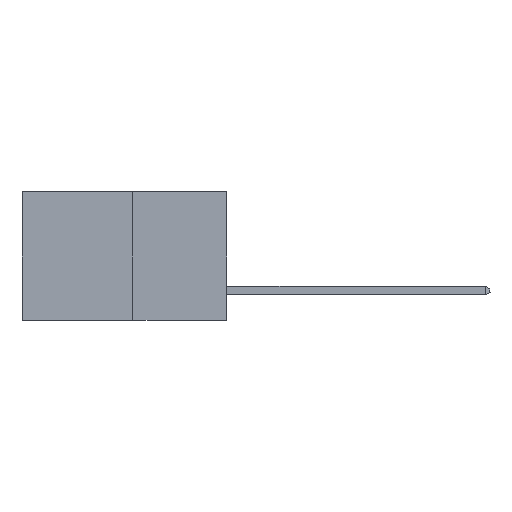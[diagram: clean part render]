
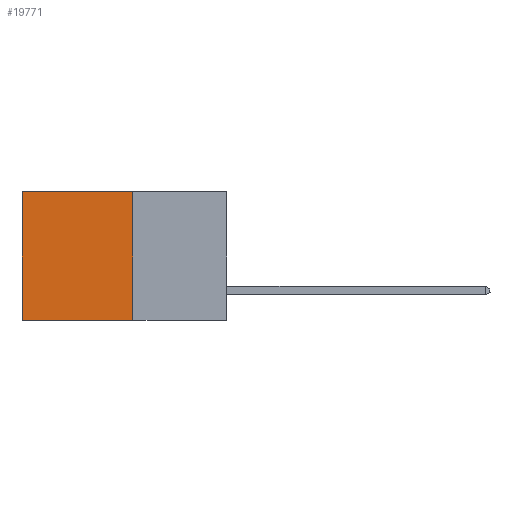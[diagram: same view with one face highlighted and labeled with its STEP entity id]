
A CAD part, left-side view. The second image highlights one B-rep face of the part: STEP entity #19771.
In plain terms, the highlighted planar face has unit normal (-1, 0, 0).
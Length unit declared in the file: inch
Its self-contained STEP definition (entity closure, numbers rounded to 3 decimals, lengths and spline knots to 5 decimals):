
#336 = EDGE_CURVE ( 'NONE', #10255, #24896, #18124, .T. ) ;
#1168 = EDGE_CURVE ( 'NONE', #4737, #10255, #10247, .T. ) ;
#2337 = CARTESIAN_POINT ( 'NONE',  ( 0.277, 0.59, 0. ) ) ;
#2595 = EDGE_CURVE ( 'NONE', #4737, #15701, #15443, .T. ) ;
#3167 = VECTOR ( 'NONE', #24520, 39.37008 ) ;
#3870 = LINE ( 'NONE', #15518, #3167 ) ;
#4200 = CARTESIAN_POINT ( 'NONE',  ( 0.277, 0.59, -0.37 ) ) ;
#4737 = VERTEX_POINT ( 'NONE', #5596 ) ;
#5028 = DIRECTION ( 'NONE',  ( 0., 1., 0. ) ) ;
#5182 = CARTESIAN_POINT ( 'NONE',  ( 0.277, 0.27, -0.37 ) ) ;
#5596 = CARTESIAN_POINT ( 'NONE',  ( 0.277, 0.27, 0. ) ) ;
#7398 = DIRECTION ( 'NONE',  ( 0., 0., -1. ) ) ;
#8435 = CARTESIAN_POINT ( 'NONE',  ( 0.277, 0.59, -0.37 ) ) ;
#9461 = VECTOR ( 'NONE', #16624, 39.37008 ) ;
#10025 = AXIS2_PLACEMENT_3D ( 'NONE', #5182, #20861, #7398 ) ;
#10247 = LINE ( 'NONE', #17994, #28091 ) ;
#10255 = VERTEX_POINT ( 'NONE', #2337 ) ;
#11436 = VECTOR ( 'NONE', #26045, 39.37008 ) ;
#13167 = ORIENTED_EDGE ( 'NONE', *, *, #1168, .T. ) ;
#15443 = LINE ( 'NONE', #15615, #9461 ) ;
#15518 = CARTESIAN_POINT ( 'NONE',  ( 0.277, 0.27, -0.37 ) ) ;
#15615 = CARTESIAN_POINT ( 'NONE',  ( 0.277, 0.27, -0.37 ) ) ;
#15701 = VERTEX_POINT ( 'NONE', #15798 ) ;
#15798 = CARTESIAN_POINT ( 'NONE',  ( 0.277, 0.27, -0.37 ) ) ;
#16102 = ORIENTED_EDGE ( 'NONE', *, *, #20894, .F. ) ;
#16346 = PLANE ( 'NONE',  #10025 ) ;
#16624 = DIRECTION ( 'NONE',  ( 0., 0., -1. ) ) ;
#17291 = EDGE_LOOP ( 'NONE', ( #28431, #16102, #17677, #13167 ) ) ;
#17677 = ORIENTED_EDGE ( 'NONE', *, *, #2595, .F. ) ;
#17994 = CARTESIAN_POINT ( 'NONE',  ( 0.277, 0.27, 0. ) ) ;
#18124 = LINE ( 'NONE', #8435, #11436 ) ;
#19771 = ADVANCED_FACE ( 'NONE', ( #22877 ), #16346, .F. ) ;
#20861 = DIRECTION ( 'NONE',  ( 1., 0., 0. ) ) ;
#20894 = EDGE_CURVE ( 'NONE', #15701, #24896, #3870, .T. ) ;
#22877 = FACE_OUTER_BOUND ( 'NONE', #17291, .T. ) ;
#24520 = DIRECTION ( 'NONE',  ( 0., 1., 0. ) ) ;
#24896 = VERTEX_POINT ( 'NONE', #4200 ) ;
#26045 = DIRECTION ( 'NONE',  ( 0., 0., -1. ) ) ;
#28091 = VECTOR ( 'NONE', #5028, 39.37008 ) ;
#28431 = ORIENTED_EDGE ( 'NONE', *, *, #336, .T. ) ;
